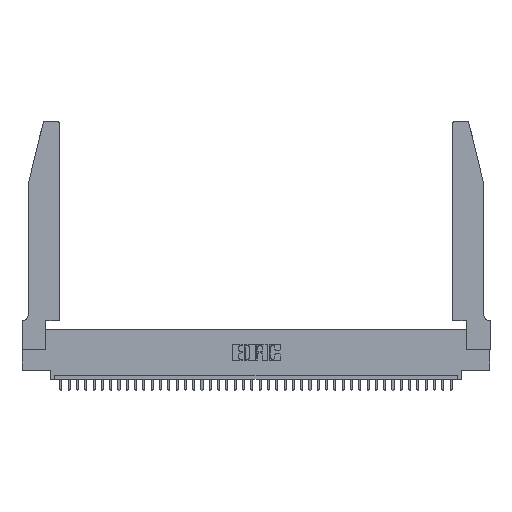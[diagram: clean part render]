
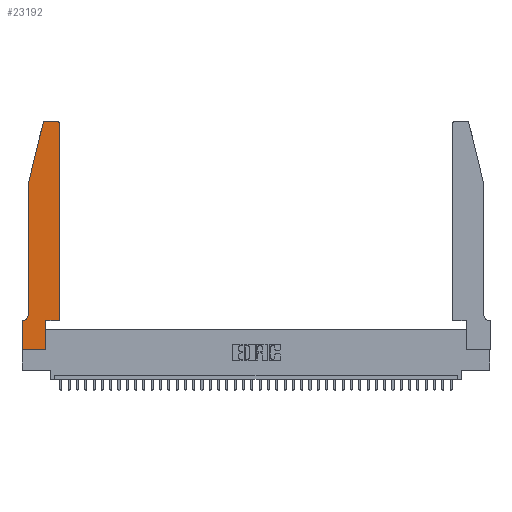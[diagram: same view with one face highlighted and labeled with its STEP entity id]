
A CAD part, top view. The second image highlights one B-rep face of the part: STEP entity #23192.
In plain terms, the highlighted planar face has unit normal (0, 0, 1).
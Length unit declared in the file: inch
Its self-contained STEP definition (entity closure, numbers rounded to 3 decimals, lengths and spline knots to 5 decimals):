
#144 = LINE ( 'NONE', #38444, #40052 ) ;
#844 = VERTEX_POINT ( 'NONE', #2354 ) ;
#872 = VERTEX_POINT ( 'NONE', #30341 ) ;
#1856 = VERTEX_POINT ( 'NONE', #10339 ) ;
#1870 = CIRCLE ( 'NONE', #24268, 0.03 ) ;
#2354 = CARTESIAN_POINT ( 'NONE',  ( 0.4505, 0.35, 0.37 ) ) ;
#2849 = DIRECTION ( 'NONE',  ( 0., -1., 0. ) ) ;
#3381 = LINE ( 'NONE', #16404, #15593 ) ;
#3659 = EDGE_CURVE ( 'NONE', #19001, #37391, #1870, .T. ) ;
#3750 = DIRECTION ( 'NONE',  ( 1., 0., 0. ) ) ;
#4551 = AXIS2_PLACEMENT_3D ( 'NONE', #28257, #6650, #16072 ) ;
#4665 = EDGE_CURVE ( 'NONE', #37391, #7721, #34642, .T. ) ;
#5413 = EDGE_CURVE ( 'NONE', #29630, #19001, #18620, .T. ) ;
#5572 = LINE ( 'NONE', #19423, #39105 ) ;
#5979 = VECTOR ( 'NONE', #35926, 39.37008 ) ;
#6650 = DIRECTION ( 'NONE',  ( 0., 0., -1. ) ) ;
#6772 = DIRECTION ( 'NONE',  ( 0., 0., 1. ) ) ;
#7668 = CARTESIAN_POINT ( 'NONE',  ( 0.0755, 0.35, 0.37 ) ) ;
#7721 = VERTEX_POINT ( 'NONE', #38072 ) ;
#8183 = DIRECTION ( 'NONE',  ( 1., 0., 0. ) ) ;
#8651 = AXIS2_PLACEMENT_3D ( 'NONE', #25570, #13091, #26578 ) ;
#8726 = CARTESIAN_POINT ( 'NONE',  ( 0.2865, 0.35, 0.37 ) ) ;
#8789 = EDGE_CURVE ( 'NONE', #7721, #26157, #33916, .T. ) ;
#8953 = DIRECTION ( 'NONE',  ( 0., 1., 0. ) ) ;
#9559 = VECTOR ( 'NONE', #8953, 39.37008 ) ;
#10151 = CARTESIAN_POINT ( 'NONE',  ( 0.284, 2.75, 0.37 ) ) ;
#10233 = EDGE_CURVE ( 'NONE', #844, #872, #5572, .T. ) ;
#10274 = VECTOR ( 'NONE', #28811, 39.37008 ) ;
#10339 = CARTESIAN_POINT ( 'NONE',  ( 0.2865, 0., 0.37 ) ) ;
#10818 = ORIENTED_EDGE ( 'NONE', *, *, #3659, .T. ) ;
#10964 = ORIENTED_EDGE ( 'NONE', *, *, #8789, .T. ) ;
#11873 = CARTESIAN_POINT ( 'NONE',  ( 0.284, 2.72, 0.37 ) ) ;
#12006 = VECTOR ( 'NONE', #3750, 39.37008 ) ;
#12285 = CIRCLE ( 'NONE', #4551, 0.07 ) ;
#12312 = CARTESIAN_POINT ( 'NONE',  ( 0.4205, 2.75, 0.37 ) ) ;
#12318 = CARTESIAN_POINT ( 'NONE',  ( 0.25487, 2.72718, 0.37 ) ) ;
#12551 = EDGE_CURVE ( 'NONE', #1856, #36654, #22723, .T. ) ;
#13028 = ORIENTED_EDGE ( 'NONE', *, *, #5413, .T. ) ;
#13076 = ORIENTED_EDGE ( 'NONE', *, *, #31684, .T. ) ;
#13091 = DIRECTION ( 'NONE',  ( 0., 0., 1. ) ) ;
#13432 = CARTESIAN_POINT ( 'NONE',  ( 0.4505, 0.35, 0.37 ) ) ;
#13899 = EDGE_CURVE ( 'NONE', #34162, #1856, #144, .T. ) ;
#14767 = EDGE_CURVE ( 'NONE', #35271, #34487, #17730, .T. ) ;
#14865 = ORIENTED_EDGE ( 'NONE', *, *, #13899, .T. ) ;
#15542 = PLANE ( 'NONE',  #36634 ) ;
#15593 = VECTOR ( 'NONE', #29147, 39.37008 ) ;
#15913 = EDGE_LOOP ( 'NONE', ( #13028, #10818, #18075, #10964, #13076, #23141, #18095, #14865, #16162, #37482, #39967, #30195 ) ) ;
#16072 = DIRECTION ( 'NONE',  ( -1., 0., 0. ) ) ;
#16096 = EDGE_CURVE ( 'NONE', #34487, #34162, #3381, .T. ) ;
#16162 = ORIENTED_EDGE ( 'NONE', *, *, #12551, .T. ) ;
#16404 = CARTESIAN_POINT ( 'NONE',  ( 0., 0., 0.37 ) ) ;
#17730 = LINE ( 'NONE', #7668, #5979 ) ;
#17818 = FACE_OUTER_BOUND ( 'NONE', #15913, .T. ) ;
#18075 = ORIENTED_EDGE ( 'NONE', *, *, #4665, .T. ) ;
#18095 = ORIENTED_EDGE ( 'NONE', *, *, #16096, .T. ) ;
#18197 = VECTOR ( 'NONE', #19663, 39.37008 ) ;
#18620 = LINE ( 'NONE', #34031, #10274 ) ;
#19001 = VERTEX_POINT ( 'NONE', #10151 ) ;
#19074 = EDGE_CURVE ( 'NONE', #36654, #844, #27042, .T. ) ;
#19335 = VECTOR ( 'NONE', #2849, 39.37008 ) ;
#19423 = CARTESIAN_POINT ( 'NONE',  ( 0.4505, 0.35, 0.37 ) ) ;
#19663 = DIRECTION ( 'NONE',  ( -0.239, -0.971, 0. ) ) ;
#22723 = LINE ( 'NONE', #29252, #9559 ) ;
#23141 = ORIENTED_EDGE ( 'NONE', *, *, #14767, .T. ) ;
#23192 = ADVANCED_FACE ( 'NONE', ( #17818 ), #15542, .T. ) ;
#23813 = CIRCLE ( 'NONE', #8651, 0.03 ) ;
#24023 = CARTESIAN_POINT ( 'NONE',  ( 0., 0.35, 0.37 ) ) ;
#24268 = AXIS2_PLACEMENT_3D ( 'NONE', #11873, #26953, #30073 ) ;
#25570 = CARTESIAN_POINT ( 'NONE',  ( 0.4205, 2.72, 0.37 ) ) ;
#26157 = VERTEX_POINT ( 'NONE', #36091 ) ;
#26578 = DIRECTION ( 'NONE',  ( 1., 0., 0. ) ) ;
#26953 = DIRECTION ( 'NONE',  ( 0., 0., 1. ) ) ;
#27042 = LINE ( 'NONE', #13432, #12006 ) ;
#28257 = CARTESIAN_POINT ( 'NONE',  ( 0.0055, 0.42, 0.37 ) ) ;
#28811 = DIRECTION ( 'NONE',  ( -1., 0., 0. ) ) ;
#29147 = DIRECTION ( 'NONE',  ( 0., -1., 0. ) ) ;
#29252 = CARTESIAN_POINT ( 'NONE',  ( 0.2865, 0.35, 0.37 ) ) ;
#29630 = VERTEX_POINT ( 'NONE', #12312 ) ;
#30073 = DIRECTION ( 'NONE',  ( 1., 0., 0. ) ) ;
#30195 = ORIENTED_EDGE ( 'NONE', *, *, #37513, .T. ) ;
#30341 = CARTESIAN_POINT ( 'NONE',  ( 0.4505, 2.72, 0.37 ) ) ;
#31118 = CARTESIAN_POINT ( 'NONE',  ( 0., 0.35, 0.37 ) ) ;
#31238 = DIRECTION ( 'NONE',  ( 1., 0., 0. ) ) ;
#31684 = EDGE_CURVE ( 'NONE', #26157, #35271, #12285, .T. ) ;
#31953 = CARTESIAN_POINT ( 'NONE',  ( 0.0755, 2., 0.37 ) ) ;
#33916 = LINE ( 'NONE', #38490, #19335 ) ;
#34031 = CARTESIAN_POINT ( 'NONE',  ( 0.2605, 2.75, 0.37 ) ) ;
#34162 = VERTEX_POINT ( 'NONE', #37454 ) ;
#34487 = VERTEX_POINT ( 'NONE', #24023 ) ;
#34642 = LINE ( 'NONE', #31953, #18197 ) ;
#35271 = VERTEX_POINT ( 'NONE', #36134 ) ;
#35926 = DIRECTION ( 'NONE',  ( -1., 0., 0. ) ) ;
#36091 = CARTESIAN_POINT ( 'NONE',  ( 0.0755, 0.42, 0.37 ) ) ;
#36134 = CARTESIAN_POINT ( 'NONE',  ( 0.0055, 0.35, 0.37 ) ) ;
#36634 = AXIS2_PLACEMENT_3D ( 'NONE', #31118, #6772, #31238 ) ;
#36654 = VERTEX_POINT ( 'NONE', #8726 ) ;
#37391 = VERTEX_POINT ( 'NONE', #12318 ) ;
#37454 = CARTESIAN_POINT ( 'NONE',  ( 0., 0., 0.37 ) ) ;
#37482 = ORIENTED_EDGE ( 'NONE', *, *, #19074, .T. ) ;
#37513 = EDGE_CURVE ( 'NONE', #872, #29630, #23813, .T. ) ;
#38072 = CARTESIAN_POINT ( 'NONE',  ( 0.0755, 2., 0.37 ) ) ;
#38444 = CARTESIAN_POINT ( 'NONE',  ( 0., 0., 0.37 ) ) ;
#38490 = CARTESIAN_POINT ( 'NONE',  ( 0.0755, 2., 0.37 ) ) ;
#38672 = DIRECTION ( 'NONE',  ( 0., 1., 0. ) ) ;
#39105 = VECTOR ( 'NONE', #38672, 39.37008 ) ;
#39967 = ORIENTED_EDGE ( 'NONE', *, *, #10233, .T. ) ;
#40052 = VECTOR ( 'NONE', #8183, 39.37008 ) ;
